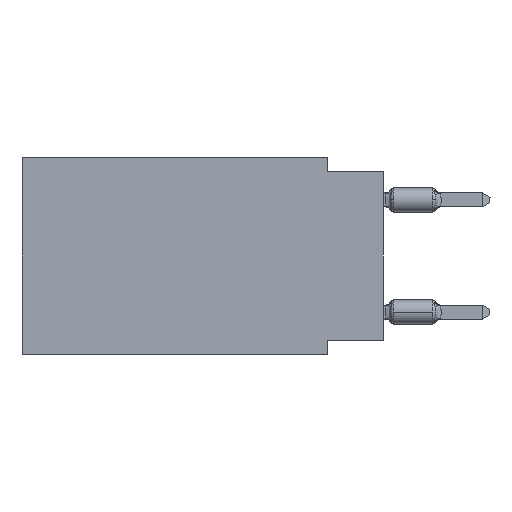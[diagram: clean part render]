
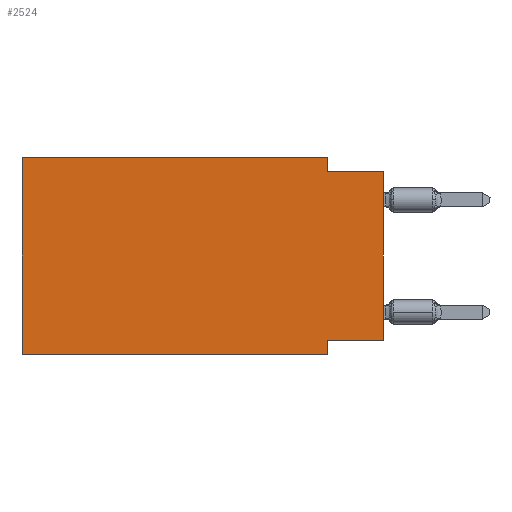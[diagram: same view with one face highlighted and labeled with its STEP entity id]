
A CAD part, left-side view. The second image highlights one B-rep face of the part: STEP entity #2524.
In plain terms, the highlighted planar face has unit normal (-1, 0, 0).
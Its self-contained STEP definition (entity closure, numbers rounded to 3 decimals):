
#947 = VERTEX_POINT ( 'NONE', #6885 ) ;
#2524 = ADVANCED_FACE ( 'NONE', ( #42950 ), #52463, .F. ) ;
#4954 = VECTOR ( 'NONE', #17536, 1000. ) ;
#6885 = CARTESIAN_POINT ( 'NONE',  ( 0., 2.54, -8.255 ) ) ;
#7081 = DIRECTION ( 'NONE',  ( 0., 0., -1. ) ) ;
#8620 = CARTESIAN_POINT ( 'NONE',  ( 0., 2.54, 0. ) ) ;
#8819 = ORIENTED_EDGE ( 'NONE', *, *, #22386, .F. ) ;
#11245 = CARTESIAN_POINT ( 'NONE',  ( 0., 2.54, -0.635 ) ) ;
#11614 = LINE ( 'NONE', #42026, #29781 ) ;
#13592 = VECTOR ( 'NONE', #47052, 1000. ) ;
#13660 = DIRECTION ( 'NONE',  ( 0., 0., 1. ) ) ;
#15405 = VECTOR ( 'NONE', #41796, 1000. ) ;
#16018 = VECTOR ( 'NONE', #34512, 1000. ) ;
#16093 = VECTOR ( 'NONE', #22167, 1000. ) ;
#16346 = CARTESIAN_POINT ( 'NONE',  ( 0., 0., -8.255 ) ) ;
#16840 = EDGE_CURVE ( 'NONE', #41241, #21714, #24798, .T. ) ;
#17454 = ORIENTED_EDGE ( 'NONE', *, *, #17639, .F. ) ;
#17536 = DIRECTION ( 'NONE',  ( 0., -1., 0. ) ) ;
#17639 = EDGE_CURVE ( 'NONE', #947, #21714, #36390, .T. ) ;
#18628 = VERTEX_POINT ( 'NONE', #8620 ) ;
#20165 = ORIENTED_EDGE ( 'NONE', *, *, #26121, .F. ) ;
#21714 = VERTEX_POINT ( 'NONE', #51738 ) ;
#22167 = DIRECTION ( 'NONE',  ( 0., -1., 0. ) ) ;
#22386 = EDGE_CURVE ( 'NONE', #34491, #947, #25283, .T. ) ;
#22474 = EDGE_LOOP ( 'NONE', ( #42862, #29581, #43735, #37757, #20165, #33651, #17454, #8819 ) ) ;
#22587 = VECTOR ( 'NONE', #13660, 1000. ) ;
#22750 = CARTESIAN_POINT ( 'NONE',  ( 0., 2.54, 0. ) ) ;
#22991 = VERTEX_POINT ( 'NONE', #42784 ) ;
#23688 = VECTOR ( 'NONE', #7081, 1000. ) ;
#24798 = LINE ( 'NONE', #37624, #4954 ) ;
#25283 = LINE ( 'NONE', #16346, #13592 ) ;
#26121 = EDGE_CURVE ( 'NONE', #41241, #22991, #11614, .T. ) ;
#27497 = EDGE_CURVE ( 'NONE', #18628, #37936, #31385, .T. ) ;
#28563 = AXIS2_PLACEMENT_3D ( 'NONE', #35656, #35134, #43772 ) ;
#29581 = ORIENTED_EDGE ( 'NONE', *, *, #53464, .F. ) ;
#29781 = VECTOR ( 'NONE', #54359, 1000. ) ;
#31385 = LINE ( 'NONE', #22750, #16018 ) ;
#33651 = ORIENTED_EDGE ( 'NONE', *, *, #16840, .T. ) ;
#33714 = CARTESIAN_POINT ( 'NONE',  ( 0., 16.383, 0. ) ) ;
#34491 = VERTEX_POINT ( 'NONE', #48997 ) ;
#34512 = DIRECTION ( 'NONE',  ( 0., 0., -1. ) ) ;
#34867 = LINE ( 'NONE', #51923, #22587 ) ;
#35134 = DIRECTION ( 'NONE',  ( 1., 0., 0. ) ) ;
#35656 = CARTESIAN_POINT ( 'NONE',  ( 0., 16.383, 0. ) ) ;
#36390 = LINE ( 'NONE', #54295, #23688 ) ;
#37118 = CARTESIAN_POINT ( 'NONE',  ( 0., 0., -0.635 ) ) ;
#37624 = CARTESIAN_POINT ( 'NONE',  ( 0., 16.383, -8.89 ) ) ;
#37757 = ORIENTED_EDGE ( 'NONE', *, *, #44398, .F. ) ;
#37936 = VERTEX_POINT ( 'NONE', #11245 ) ;
#41241 = VERTEX_POINT ( 'NONE', #47777 ) ;
#41796 = DIRECTION ( 'NONE',  ( 0., -1., 0. ) ) ;
#42026 = CARTESIAN_POINT ( 'NONE',  ( 0., 16.383, 0. ) ) ;
#42784 = CARTESIAN_POINT ( 'NONE',  ( 0., 16.383, 0. ) ) ;
#42862 = ORIENTED_EDGE ( 'NONE', *, *, #43027, .T. ) ;
#42950 = FACE_OUTER_BOUND ( 'NONE', #22474, .T. ) ;
#43027 = EDGE_CURVE ( 'NONE', #34491, #55130, #34867, .T. ) ;
#43370 = CARTESIAN_POINT ( 'NONE',  ( 0., 0., -0.635 ) ) ;
#43735 = ORIENTED_EDGE ( 'NONE', *, *, #27497, .F. ) ;
#43772 = DIRECTION ( 'NONE',  ( 0., 0., -1. ) ) ;
#44180 = LINE ( 'NONE', #43370, #16093 ) ;
#44398 = EDGE_CURVE ( 'NONE', #22991, #18628, #49914, .T. ) ;
#47052 = DIRECTION ( 'NONE',  ( 0., 1., 0. ) ) ;
#47777 = CARTESIAN_POINT ( 'NONE',  ( 0., 16.383, -8.89 ) ) ;
#48997 = CARTESIAN_POINT ( 'NONE',  ( 0., 0., -8.255 ) ) ;
#49914 = LINE ( 'NONE', #33714, #15405 ) ;
#51738 = CARTESIAN_POINT ( 'NONE',  ( 0., 2.54, -8.89 ) ) ;
#51923 = CARTESIAN_POINT ( 'NONE',  ( 0., 0., 0. ) ) ;
#52463 = PLANE ( 'NONE',  #28563 ) ;
#53464 = EDGE_CURVE ( 'NONE', #37936, #55130, #44180, .T. ) ;
#54295 = CARTESIAN_POINT ( 'NONE',  ( 0., 2.54, -8.89 ) ) ;
#54359 = DIRECTION ( 'NONE',  ( 0., 0., 1. ) ) ;
#55130 = VERTEX_POINT ( 'NONE', #37118 ) ;
